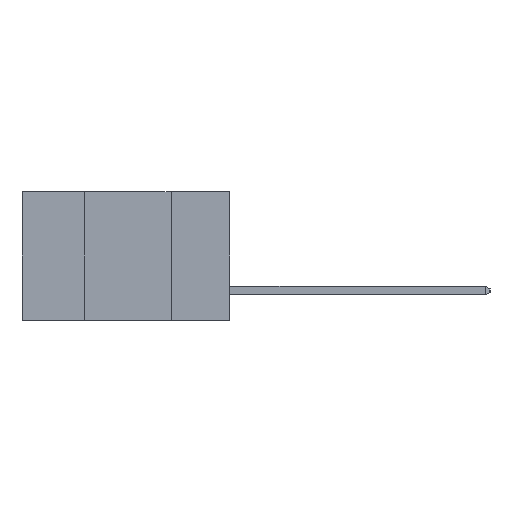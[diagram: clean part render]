
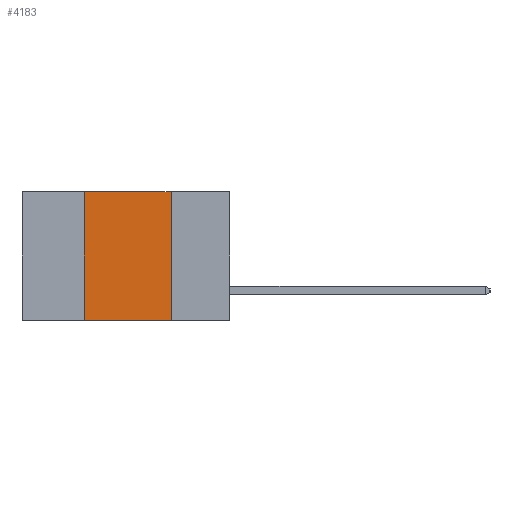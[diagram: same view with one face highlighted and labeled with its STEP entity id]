
A CAD part, left-side view. The second image highlights one B-rep face of the part: STEP entity #4183.
In plain terms, the highlighted planar face has unit normal (-1, 0, 0).
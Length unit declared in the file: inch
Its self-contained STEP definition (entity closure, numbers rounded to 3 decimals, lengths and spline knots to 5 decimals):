
#78 = CARTESIAN_POINT ( 'NONE',  ( 0., 0.17, 0. ) ) ;
#162 = ORIENTED_EDGE ( 'NONE', *, *, #4431, .F. ) ;
#213 = EDGE_CURVE ( 'NONE', #8791, #571, #551, .T. ) ;
#551 = LINE ( 'NONE', #6890, #4736 ) ;
#571 = VERTEX_POINT ( 'NONE', #2472 ) ;
#660 = VERTEX_POINT ( 'NONE', #9458 ) ;
#1655 = DIRECTION ( 'NONE',  ( 1., 0., 0. ) ) ;
#1973 = ORIENTED_EDGE ( 'NONE', *, *, #2926, .F. ) ;
#2472 = CARTESIAN_POINT ( 'NONE',  ( 0., 0.42, 0. ) ) ;
#2606 = DIRECTION ( 'NONE',  ( 0., 0., -1. ) ) ;
#2809 = PLANE ( 'NONE',  #9199 ) ;
#2838 = VECTOR ( 'NONE', #6133, 39.37008 ) ;
#2926 = EDGE_CURVE ( 'NONE', #6139, #660, #10283, .T. ) ;
#3119 = EDGE_LOOP ( 'NONE', ( #1973, #162, #7974, #8301 ) ) ;
#3556 = LINE ( 'NONE', #8242, #7585 ) ;
#4183 = ADVANCED_FACE ( 'NONE', ( #5941 ), #2809, .F. ) ;
#4431 = EDGE_CURVE ( 'NONE', #571, #6139, #7643, .T. ) ;
#4736 = VECTOR ( 'NONE', #7639, 39.37008 ) ;
#5796 = CARTESIAN_POINT ( 'NONE',  ( 0., 0.6, 0. ) ) ;
#5941 = FACE_OUTER_BOUND ( 'NONE', #3119, .T. ) ;
#6133 = DIRECTION ( 'NONE',  ( 0., -1., 0. ) ) ;
#6139 = VERTEX_POINT ( 'NONE', #78 ) ;
#6202 = EDGE_CURVE ( 'NONE', #8791, #660, #3556, .T. ) ;
#6337 = VECTOR ( 'NONE', #7556, 39.37008 ) ;
#6890 = CARTESIAN_POINT ( 'NONE',  ( 0., 0.42, 0. ) ) ;
#7556 = DIRECTION ( 'NONE',  ( 0., 0., -1. ) ) ;
#7585 = VECTOR ( 'NONE', #8258, 39.37008 ) ;
#7639 = DIRECTION ( 'NONE',  ( 0., 0., 1. ) ) ;
#7643 = LINE ( 'NONE', #8303, #2838 ) ;
#7766 = CARTESIAN_POINT ( 'NONE',  ( 0., 0.17, 0. ) ) ;
#7974 = ORIENTED_EDGE ( 'NONE', *, *, #213, .F. ) ;
#8242 = CARTESIAN_POINT ( 'NONE',  ( 0., 0.6, -0.37 ) ) ;
#8258 = DIRECTION ( 'NONE',  ( 0., -1., 0. ) ) ;
#8301 = ORIENTED_EDGE ( 'NONE', *, *, #6202, .T. ) ;
#8303 = CARTESIAN_POINT ( 'NONE',  ( 0., 0.6, 0. ) ) ;
#8791 = VERTEX_POINT ( 'NONE', #9616 ) ;
#9199 = AXIS2_PLACEMENT_3D ( 'NONE', #5796, #1655, #2606 ) ;
#9458 = CARTESIAN_POINT ( 'NONE',  ( 0., 0.17, -0.37 ) ) ;
#9616 = CARTESIAN_POINT ( 'NONE',  ( 0., 0.42, -0.37 ) ) ;
#10283 = LINE ( 'NONE', #7766, #6337 ) ;
